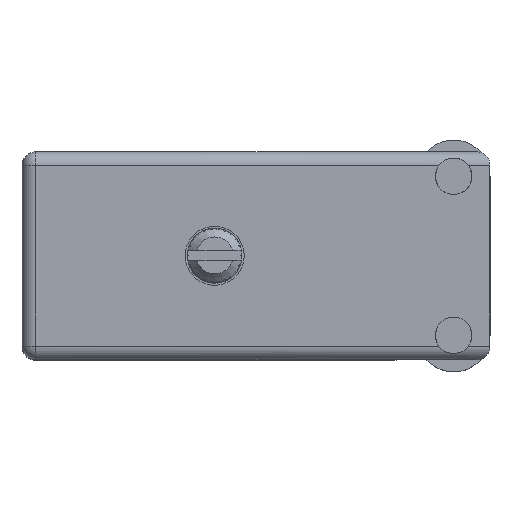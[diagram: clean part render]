
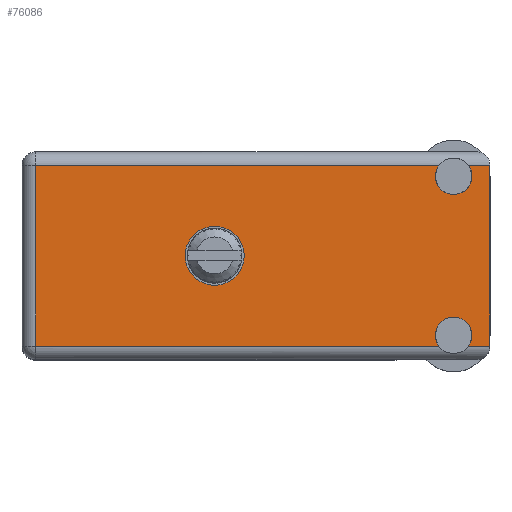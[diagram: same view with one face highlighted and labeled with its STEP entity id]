
A CAD part, top view. The second image highlights one B-rep face of the part: STEP entity #76086.
In plain terms, the highlighted face is planar.
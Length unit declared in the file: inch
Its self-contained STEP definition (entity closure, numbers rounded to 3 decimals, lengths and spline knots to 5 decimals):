
#785 = EDGE_CURVE ( 'NONE', #16953, #109306, #112156, .T. ) ;
#1160 = CARTESIAN_POINT ( 'NONE',  ( 1.484, 0.906, -0.5685 ) ) ;
#4586 = CIRCLE ( 'NONE', #191073, 0.0625 ) ;
#4931 = EDGE_CURVE ( 'NONE', #18016, #98705, #78674, .T. ) ;
#10278 = ORIENTED_EDGE ( 'NONE', *, *, #112288, .F. ) ;
#11572 = ORIENTED_EDGE ( 'NONE', *, *, #28383, .F. ) ;
#12159 = EDGE_CURVE ( 'NONE', #148663, #28818, #67957, .T. ) ;
#12743 = VECTOR ( 'NONE', #31440, 39.37008 ) ;
#16165 = CARTESIAN_POINT ( 'NONE',  ( 1.53437, 0.906, -0.668 ) ) ;
#16953 = VERTEX_POINT ( 'NONE', #184797 ) ;
#18016 = VERTEX_POINT ( 'NONE', #54165 ) ;
#19668 = EDGE_CURVE ( 'NONE', #86137, #28818, #49480, .T. ) ;
#20125 = CIRCLE ( 'NONE', #37802, 0.0625 ) ;
#26308 = ORIENTED_EDGE ( 'NONE', *, *, #153553, .T. ) ;
#26769 = DIRECTION ( 'NONE',  ( 0., 1., 0. ) ) ;
#28383 = EDGE_CURVE ( 'NONE', #165293, #148663, #20125, .T. ) ;
#28818 = VERTEX_POINT ( 'NONE', #16165 ) ;
#30611 = DIRECTION ( 'NONE',  ( 0., 0., 1. ) ) ;
#31440 = DIRECTION ( 'NONE',  ( 0., 0., 1. ) ) ;
#31923 = ORIENTED_EDGE ( 'NONE', *, *, #148379, .F. ) ;
#37413 = DIRECTION ( 'NONE',  ( 1., 0., 0. ) ) ;
#37802 = AXIS2_PLACEMENT_3D ( 'NONE', #105979, #59838, #134421 ) ;
#39139 = DIRECTION ( 'NONE',  ( 0., 0., 1. ) ) ;
#40746 = DIRECTION ( 'NONE',  ( 0., 1., 0. ) ) ;
#40852 = CARTESIAN_POINT ( 'NONE',  ( 0., 0.906, -0.668 ) ) ;
#41092 = ORIENTED_EDGE ( 'NONE', *, *, #106544, .F. ) ;
#41358 = DIRECTION ( 'NONE',  ( -1., 0., 0. ) ) ;
#42008 = VECTOR ( 'NONE', #39139, 39.37008 ) ;
#42569 = CARTESIAN_POINT ( 'NONE',  ( 1.484, 0.906, -0.084 ) ) ;
#45807 = VECTOR ( 'NONE', #37413, 39.37008 ) ;
#45843 = AXIS2_PLACEMENT_3D ( 'NONE', #167797, #74714, #30611 ) ;
#48548 = ORIENTED_EDGE ( 'NONE', *, *, #785, .F. ) ;
#49480 = LINE ( 'NONE', #40852, #132229 ) ;
#51238 = CARTESIAN_POINT ( 'NONE',  ( 1.609, 0.906, -0.047 ) ) ;
#54165 = CARTESIAN_POINT ( 'NONE',  ( 0.047, 0.906, -0.668 ) ) ;
#55182 = CARTESIAN_POINT ( 'NONE',  ( 0.6625, 0.906, -0.3575 ) ) ;
#59838 = DIRECTION ( 'NONE',  ( 0., 1., 0. ) ) ;
#61036 = VERTEX_POINT ( 'NONE', #85626 ) ;
#66781 = CARTESIAN_POINT ( 'NONE',  ( 1.484, 0.906, -0.631 ) ) ;
#67957 = CIRCLE ( 'NONE', #144734, 0.0625 ) ;
#68613 = ORIENTED_EDGE ( 'NONE', *, *, #19668, .T. ) ;
#73904 = LINE ( 'NONE', #102546, #173237 ) ;
#74714 = DIRECTION ( 'NONE',  ( 0., 1., 0. ) ) ;
#74733 = VERTEX_POINT ( 'NONE', #91807 ) ;
#75830 = EDGE_CURVE ( 'NONE', #165186, #74733, #142577, .T. ) ;
#76060 = EDGE_CURVE ( 'NONE', #98705, #178313, #73904, .T. ) ;
#76086 = ADVANCED_FACE ( 'NONE', ( #126134, #149520 ), #132320, .T. ) ;
#76283 = ORIENTED_EDGE ( 'NONE', *, *, #76060, .T. ) ;
#78674 = LINE ( 'NONE', #193745, #12743 ) ;
#80621 = DIRECTION ( 'NONE',  ( 0., 1., 0. ) ) ;
#84219 = DIRECTION ( 'NONE',  ( 0., 0., 1. ) ) ;
#85626 = CARTESIAN_POINT ( 'NONE',  ( 1.484, 0.906, -0.1465 ) ) ;
#86137 = VERTEX_POINT ( 'NONE', #145200 ) ;
#91807 = CARTESIAN_POINT ( 'NONE',  ( 1.609, 0.906, -0.047 ) ) ;
#95202 = EDGE_CURVE ( 'NONE', #165186, #61036, #118848, .T. ) ;
#95575 = CARTESIAN_POINT ( 'NONE',  ( 0.047, 0.906, -0.047 ) ) ;
#95633 = CARTESIAN_POINT ( 'NONE',  ( 0.6625, 0.906, -0.459 ) ) ;
#98705 = VERTEX_POINT ( 'NONE', #95575 ) ;
#102546 = CARTESIAN_POINT ( 'NONE',  ( 1.609, 0.906, -0.047 ) ) ;
#105979 = CARTESIAN_POINT ( 'NONE',  ( 1.484, 0.906, -0.631 ) ) ;
#106544 = EDGE_CURVE ( 'NONE', #61036, #178313, #4586, .T. ) ;
#109306 = VERTEX_POINT ( 'NONE', #95633 ) ;
#112156 = CIRCLE ( 'NONE', #136159, 0.1015 ) ;
#112288 = EDGE_CURVE ( 'NONE', #109306, #16953, #149804, .T. ) ;
#112958 = CARTESIAN_POINT ( 'NONE',  ( 1.609, 0.906, 0. ) ) ;
#118456 = CARTESIAN_POINT ( 'NONE',  ( 0., 0.906, -0.668 ) ) ;
#118669 = CARTESIAN_POINT ( 'NONE',  ( 1.43363, 0.906, -0.668 ) ) ;
#118848 = CIRCLE ( 'NONE', #45843, 0.0625 ) ;
#119034 = EDGE_LOOP ( 'NONE', ( #48548, #10278 ) ) ;
#126134 = FACE_BOUND ( 'NONE', #119034, .T. ) ;
#132229 = VECTOR ( 'NONE', #176103, 39.37008 ) ;
#132313 = DIRECTION ( 'NONE',  ( 0., 0., 1. ) ) ;
#132320 = PLANE ( 'NONE',  #167744 ) ;
#132742 = CARTESIAN_POINT ( 'NONE',  ( 1.53437, 0.906, -0.047 ) ) ;
#134421 = DIRECTION ( 'NONE',  ( 0., 0., 1. ) ) ;
#135116 = ORIENTED_EDGE ( 'NONE', *, *, #12159, .F. ) ;
#136159 = AXIS2_PLACEMENT_3D ( 'NONE', #55182, #174640, #84219 ) ;
#140706 = CARTESIAN_POINT ( 'NONE',  ( 1.43363, 0.906, -0.047 ) ) ;
#142577 = LINE ( 'NONE', #51238, #45807 ) ;
#143349 = DIRECTION ( 'NONE',  ( 0., 0., 1. ) ) ;
#144734 = AXIS2_PLACEMENT_3D ( 'NONE', #66781, #80621, #143349 ) ;
#145200 = CARTESIAN_POINT ( 'NONE',  ( 1.609, 0.906, -0.668 ) ) ;
#147556 = CARTESIAN_POINT ( 'NONE',  ( 0.6625, 0.906, -0.3575 ) ) ;
#148379 = EDGE_CURVE ( 'NONE', #86137, #74733, #155409, .T. ) ;
#148663 = VERTEX_POINT ( 'NONE', #1160 ) ;
#149402 = DIRECTION ( 'NONE',  ( 0., 0., 1. ) ) ;
#149520 = FACE_OUTER_BOUND ( 'NONE', #177236, .T. ) ;
#149804 = CIRCLE ( 'NONE', #170568, 0.1015 ) ;
#153553 = EDGE_CURVE ( 'NONE', #165293, #18016, #181981, .T. ) ;
#155409 = LINE ( 'NONE', #112958, #42008 ) ;
#162625 = DIRECTION ( 'NONE',  ( 1., 0., 0. ) ) ;
#162710 = DIRECTION ( 'NONE',  ( 0., 0., 1. ) ) ;
#165186 = VERTEX_POINT ( 'NONE', #132742 ) ;
#165293 = VERTEX_POINT ( 'NONE', #118669 ) ;
#167744 = AXIS2_PLACEMENT_3D ( 'NONE', #194286, #177825, #149402 ) ;
#167797 = CARTESIAN_POINT ( 'NONE',  ( 1.484, 0.906, -0.084 ) ) ;
#170082 = ORIENTED_EDGE ( 'NONE', *, *, #75830, .T. ) ;
#170568 = AXIS2_PLACEMENT_3D ( 'NONE', #147556, #40746, #162710 ) ;
#173237 = VECTOR ( 'NONE', #162625, 39.37008 ) ;
#174640 = DIRECTION ( 'NONE',  ( 0., 1., 0. ) ) ;
#176103 = DIRECTION ( 'NONE',  ( -1., 0., 0. ) ) ;
#176369 = ORIENTED_EDGE ( 'NONE', *, *, #4931, .T. ) ;
#177236 = EDGE_LOOP ( 'NONE', ( #76283, #41092, #179887, #170082, #31923, #68613, #135116, #11572, #26308, #176369 ) ) ;
#177825 = DIRECTION ( 'NONE',  ( 0., 1., 0. ) ) ;
#178313 = VERTEX_POINT ( 'NONE', #140706 ) ;
#179887 = ORIENTED_EDGE ( 'NONE', *, *, #95202, .F. ) ;
#181787 = VECTOR ( 'NONE', #41358, 39.37008 ) ;
#181981 = LINE ( 'NONE', #118456, #181787 ) ;
#184797 = CARTESIAN_POINT ( 'NONE',  ( 0.6625, 0.906, -0.256 ) ) ;
#191073 = AXIS2_PLACEMENT_3D ( 'NONE', #42569, #26769, #132313 ) ;
#193745 = CARTESIAN_POINT ( 'NONE',  ( 0.047, 0.906, -0.715 ) ) ;
#194286 = CARTESIAN_POINT ( 'NONE',  ( 0., 0.906, -0.715 ) ) ;
